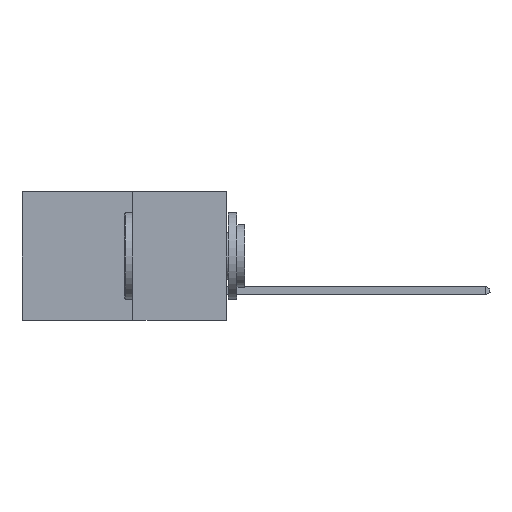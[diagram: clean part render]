
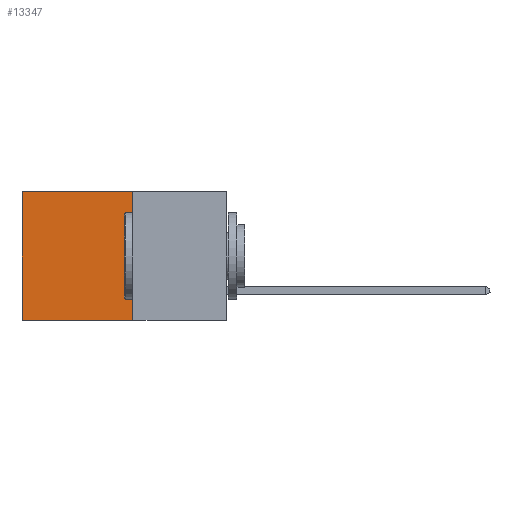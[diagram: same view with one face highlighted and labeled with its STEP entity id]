
A CAD part, left-side view. The second image highlights one B-rep face of the part: STEP entity #13347.
In plain terms, the highlighted planar face has unit normal (-1, 0, 0).
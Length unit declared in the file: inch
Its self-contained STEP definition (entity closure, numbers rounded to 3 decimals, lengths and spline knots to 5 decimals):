
#331 = EDGE_CURVE ( 'NONE', #13749, #12896, #4265, .T. ) ;
#481 = EDGE_CURVE ( 'NONE', #3093, #13749, #7500, .T. ) ;
#1660 = VERTEX_POINT ( 'NONE', #10476 ) ;
#1810 = LINE ( 'NONE', #11403, #7558 ) ;
#2751 = DIRECTION ( 'NONE',  ( 0., 0., -1. ) ) ;
#2832 = EDGE_CURVE ( 'NONE', #1660, #12896, #1810, .T. ) ;
#3093 = VERTEX_POINT ( 'NONE', #8706 ) ;
#3117 = VECTOR ( 'NONE', #8872, 39.37008 ) ;
#3252 = ORIENTED_EDGE ( 'NONE', *, *, #481, .F. ) ;
#4031 = ORIENTED_EDGE ( 'NONE', *, *, #331, .F. ) ;
#4265 = LINE ( 'NONE', #13162, #3117 ) ;
#5039 = ORIENTED_EDGE ( 'NONE', *, *, #8573, .T. ) ;
#6345 = LINE ( 'NONE', #8434, #11120 ) ;
#7500 = LINE ( 'NONE', #7725, #9578 ) ;
#7558 = VECTOR ( 'NONE', #11389, 39.37008 ) ;
#7725 = CARTESIAN_POINT ( 'NONE',  ( 0.277, 0.27, -0.37 ) ) ;
#7797 = CARTESIAN_POINT ( 'NONE',  ( 0.277, 0.27, -0.37 ) ) ;
#8313 = CARTESIAN_POINT ( 'NONE',  ( 0.277, 0.27, -0.37 ) ) ;
#8434 = CARTESIAN_POINT ( 'NONE',  ( 0.277, 0.27, 0. ) ) ;
#8505 = ORIENTED_EDGE ( 'NONE', *, *, #2832, .T. ) ;
#8573 = EDGE_CURVE ( 'NONE', #3093, #1660, #6345, .T. ) ;
#8706 = CARTESIAN_POINT ( 'NONE',  ( 0.277, 0.27, 0. ) ) ;
#8872 = DIRECTION ( 'NONE',  ( 0., 1., 0. ) ) ;
#9332 = DIRECTION ( 'NONE',  ( 1., 0., 0. ) ) ;
#9578 = VECTOR ( 'NONE', #10023, 39.37008 ) ;
#9988 = EDGE_LOOP ( 'NONE', ( #8505, #4031, #3252, #5039 ) ) ;
#10023 = DIRECTION ( 'NONE',  ( 0., 0., -1. ) ) ;
#10476 = CARTESIAN_POINT ( 'NONE',  ( 0.277, 0.59, 0. ) ) ;
#11120 = VECTOR ( 'NONE', #11916, 39.37008 ) ;
#11238 = FACE_OUTER_BOUND ( 'NONE', #9988, .T. ) ;
#11389 = DIRECTION ( 'NONE',  ( 0., 0., -1. ) ) ;
#11403 = CARTESIAN_POINT ( 'NONE',  ( 0.277, 0.59, -0.37 ) ) ;
#11916 = DIRECTION ( 'NONE',  ( 0., 1., 0. ) ) ;
#12268 = PLANE ( 'NONE',  #13556 ) ;
#12813 = CARTESIAN_POINT ( 'NONE',  ( 0.277, 0.59, -0.37 ) ) ;
#12896 = VERTEX_POINT ( 'NONE', #12813 ) ;
#13162 = CARTESIAN_POINT ( 'NONE',  ( 0.277, 0.27, -0.37 ) ) ;
#13347 = ADVANCED_FACE ( 'NONE', ( #11238 ), #12268, .F. ) ;
#13556 = AXIS2_PLACEMENT_3D ( 'NONE', #8313, #9332, #2751 ) ;
#13749 = VERTEX_POINT ( 'NONE', #7797 ) ;
